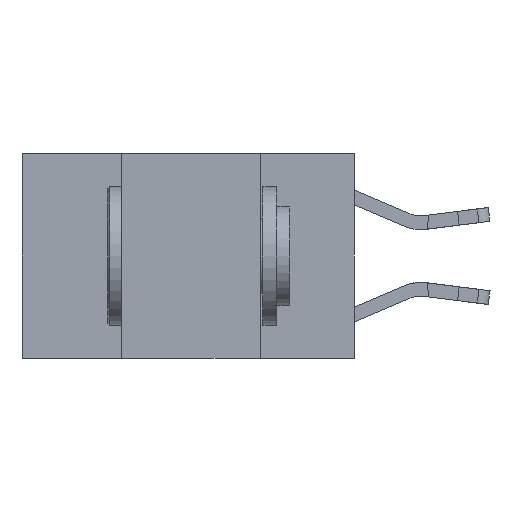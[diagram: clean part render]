
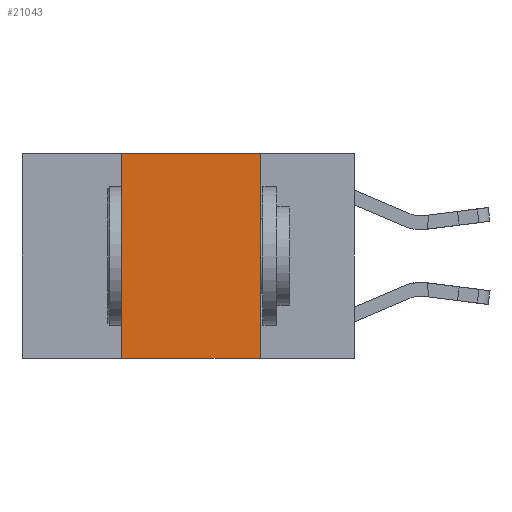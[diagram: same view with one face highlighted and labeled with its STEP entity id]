
A CAD part, left-side view. The second image highlights one B-rep face of the part: STEP entity #21043.
In plain terms, the highlighted planar face has unit normal (-1, 0, 0).
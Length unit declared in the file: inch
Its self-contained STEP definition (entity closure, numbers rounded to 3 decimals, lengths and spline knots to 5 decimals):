
#3118 = VECTOR ( 'NONE', #3274, 39.37008 ) ;
#3274 = DIRECTION ( 'NONE',  ( 0., -1., 0. ) ) ;
#3574 = ORIENTED_EDGE ( 'NONE', *, *, #4069, .F. ) ;
#4069 = EDGE_CURVE ( 'NONE', #15731, #14323, #26587, .T. ) ;
#4493 = PLANE ( 'NONE',  #18442 ) ;
#4768 = DIRECTION ( 'NONE',  ( 0., 0., -1. ) ) ;
#5661 = CARTESIAN_POINT ( 'NONE',  ( 0., 0.6, 0. ) ) ;
#6984 = LINE ( 'NONE', #23828, #18027 ) ;
#8342 = EDGE_CURVE ( 'NONE', #15894, #15731, #15644, .T. ) ;
#9554 = CARTESIAN_POINT ( 'NONE',  ( 0., 0.6, -0.37 ) ) ;
#11502 = VECTOR ( 'NONE', #16284, 39.37008 ) ;
#11778 = CARTESIAN_POINT ( 'NONE',  ( 0., 0.17, 0. ) ) ;
#11898 = EDGE_LOOP ( 'NONE', ( #3574, #13113, #20317, #17092 ) ) ;
#13113 = ORIENTED_EDGE ( 'NONE', *, *, #8342, .F. ) ;
#14323 = VERTEX_POINT ( 'NONE', #20190 ) ;
#15150 = DIRECTION ( 'NONE',  ( 1., 0., 0. ) ) ;
#15552 = LINE ( 'NONE', #9554, #3118 ) ;
#15644 = LINE ( 'NONE', #5661, #16854 ) ;
#15731 = VERTEX_POINT ( 'NONE', #20464 ) ;
#15894 = VERTEX_POINT ( 'NONE', #17169 ) ;
#16284 = DIRECTION ( 'NONE',  ( 0., 0., -1. ) ) ;
#16779 = FACE_OUTER_BOUND ( 'NONE', #11898, .T. ) ;
#16854 = VECTOR ( 'NONE', #21752, 39.37008 ) ;
#17092 = ORIENTED_EDGE ( 'NONE', *, *, #19082, .T. ) ;
#17169 = CARTESIAN_POINT ( 'NONE',  ( 0., 0.42, 0. ) ) ;
#18027 = VECTOR ( 'NONE', #24869, 39.37008 ) ;
#18442 = AXIS2_PLACEMENT_3D ( 'NONE', #20986, #15150, #4768 ) ;
#19082 = EDGE_CURVE ( 'NONE', #20874, #14323, #15552, .T. ) ;
#20190 = CARTESIAN_POINT ( 'NONE',  ( 0., 0.17, -0.37 ) ) ;
#20317 = ORIENTED_EDGE ( 'NONE', *, *, #21864, .F. ) ;
#20464 = CARTESIAN_POINT ( 'NONE',  ( 0., 0.17, 0. ) ) ;
#20874 = VERTEX_POINT ( 'NONE', #24675 ) ;
#20986 = CARTESIAN_POINT ( 'NONE',  ( 0., 0.6, 0. ) ) ;
#21043 = ADVANCED_FACE ( 'NONE', ( #16779 ), #4493, .F. ) ;
#21752 = DIRECTION ( 'NONE',  ( 0., -1., 0. ) ) ;
#21864 = EDGE_CURVE ( 'NONE', #20874, #15894, #6984, .T. ) ;
#23828 = CARTESIAN_POINT ( 'NONE',  ( 0., 0.42, 0. ) ) ;
#24675 = CARTESIAN_POINT ( 'NONE',  ( 0., 0.42, -0.37 ) ) ;
#24869 = DIRECTION ( 'NONE',  ( 0., 0., 1. ) ) ;
#26587 = LINE ( 'NONE', #11778, #11502 ) ;
